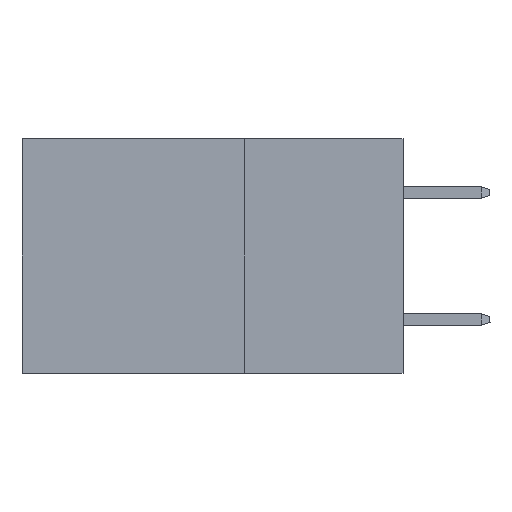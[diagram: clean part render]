
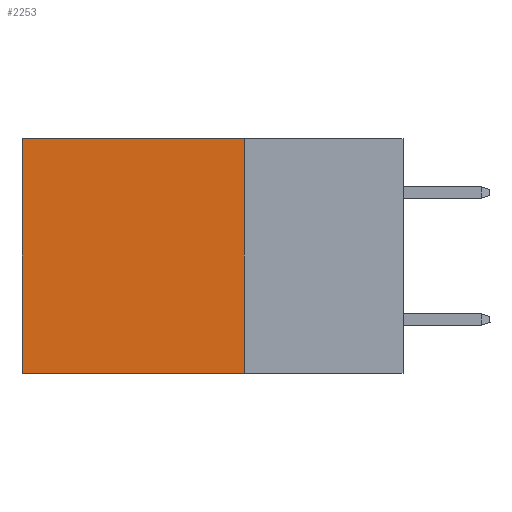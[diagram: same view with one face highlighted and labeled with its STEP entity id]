
A CAD part, left-side view. The second image highlights one B-rep face of the part: STEP entity #2253.
In plain terms, the highlighted planar face has unit normal (-1, 0, 0).
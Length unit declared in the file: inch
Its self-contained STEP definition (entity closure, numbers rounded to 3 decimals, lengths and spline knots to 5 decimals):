
#5 = VECTOR ( 'NONE', #1805, 39.37008 ) ;
#69 = PLANE ( 'NONE',  #7440 ) ;
#233 = VECTOR ( 'NONE', #9389, 39.37008 ) ;
#835 = CARTESIAN_POINT ( 'NONE',  ( 0.2875, 0.6, 0. ) ) ;
#1164 = EDGE_CURVE ( 'NONE', #9940, #9120, #5351, .T. ) ;
#1389 = EDGE_CURVE ( 'NONE', #4178, #9940, #1482, .T. ) ;
#1427 = ORIENTED_EDGE ( 'NONE', *, *, #9679, .T. ) ;
#1482 = LINE ( 'NONE', #4940, #7908 ) ;
#1625 = CARTESIAN_POINT ( 'NONE',  ( 0.2875, 0.6, 0. ) ) ;
#1805 = DIRECTION ( 'NONE',  ( 0., 1., 0. ) ) ;
#2253 = ADVANCED_FACE ( 'NONE', ( #11413 ), #69, .F. ) ;
#2970 = EDGE_LOOP ( 'NONE', ( #10465, #10432, #14607, #1427 ) ) ;
#3618 = DIRECTION ( 'NONE',  ( 1., 0., 0. ) ) ;
#3651 = CARTESIAN_POINT ( 'NONE',  ( 0.2875, 0.25, 0. ) ) ;
#4178 = VERTEX_POINT ( 'NONE', #3651 ) ;
#4360 = CARTESIAN_POINT ( 'NONE',  ( 0.2875, 0.25, 0. ) ) ;
#4368 = CARTESIAN_POINT ( 'NONE',  ( 0.2875, 0.6, -0.37 ) ) ;
#4674 = CARTESIAN_POINT ( 'NONE',  ( 0.2875, 0.25, 0. ) ) ;
#4940 = CARTESIAN_POINT ( 'NONE',  ( 0.2875, 0.25, 0. ) ) ;
#5351 = LINE ( 'NONE', #10760, #5 ) ;
#6040 = DIRECTION ( 'NONE',  ( 0., 0., -1. ) ) ;
#6862 = DIRECTION ( 'NONE',  ( 0., 1., 0. ) ) ;
#7440 = AXIS2_PLACEMENT_3D ( 'NONE', #4674, #3618, #11498 ) ;
#7585 = CARTESIAN_POINT ( 'NONE',  ( 0.2875, 0.25, -0.37 ) ) ;
#7908 = VECTOR ( 'NONE', #6040, 39.37008 ) ;
#8007 = VERTEX_POINT ( 'NONE', #835 ) ;
#9120 = VERTEX_POINT ( 'NONE', #4368 ) ;
#9389 = DIRECTION ( 'NONE',  ( 0., 0., -1. ) ) ;
#9679 = EDGE_CURVE ( 'NONE', #4178, #8007, #10127, .T. ) ;
#9940 = VERTEX_POINT ( 'NONE', #7585 ) ;
#10127 = LINE ( 'NONE', #4360, #11324 ) ;
#10432 = ORIENTED_EDGE ( 'NONE', *, *, #1164, .F. ) ;
#10465 = ORIENTED_EDGE ( 'NONE', *, *, #13936, .T. ) ;
#10760 = CARTESIAN_POINT ( 'NONE',  ( 0.2875, 0.25, -0.37 ) ) ;
#11324 = VECTOR ( 'NONE', #6862, 39.37008 ) ;
#11413 = FACE_OUTER_BOUND ( 'NONE', #2970, .T. ) ;
#11498 = DIRECTION ( 'NONE',  ( 0., 0., -1. ) ) ;
#13936 = EDGE_CURVE ( 'NONE', #8007, #9120, #13986, .T. ) ;
#13986 = LINE ( 'NONE', #1625, #233 ) ;
#14607 = ORIENTED_EDGE ( 'NONE', *, *, #1389, .F. ) ;
